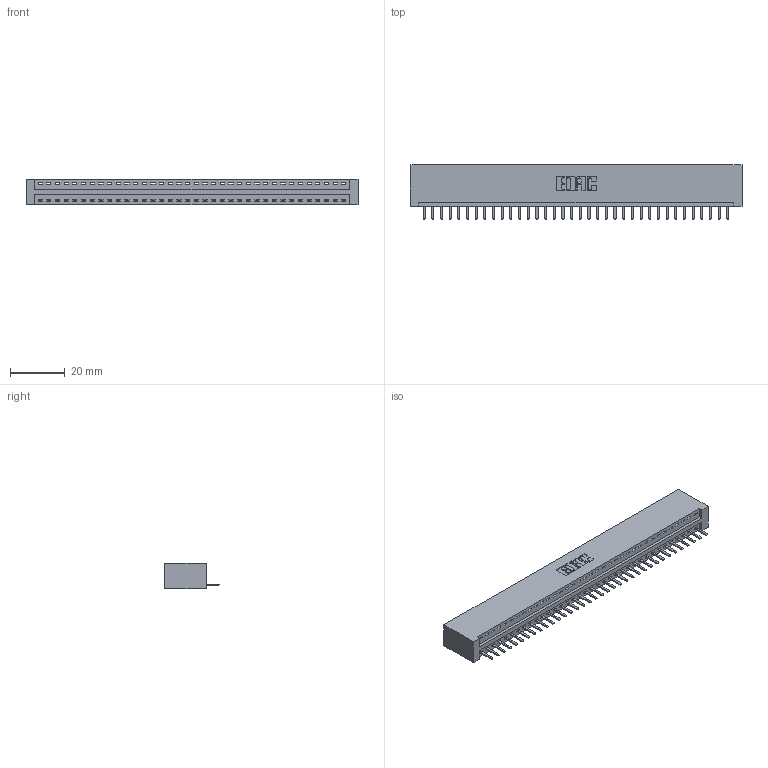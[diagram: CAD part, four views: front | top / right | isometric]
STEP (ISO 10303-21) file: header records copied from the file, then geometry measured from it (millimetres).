
FILE_DESCRIPTION (( 'STEP AP203' ), '1' );
FILE_NAME ('396-036-520-101.STEP', '2019-10-27T16:39:52', ( '' ), ( '' ), 'SwSTEP 2.0', 'SolidWorks 2016', '' );
FILE_SCHEMA (( 'CONFIG_CONTROL_DESIGN' ));
Length unit declared in the file: inch
Products named in the file (3): 346 Part_No Mounting Lugs; 396-036-520-101; 345-292-001_345-293-120
Assembly tree (37 placements, depth 2):
  396-036-520-101
    346 Part_No Mounting Lugs
    345-292-001_345-293-120  x36
Bounding box: 121.54 x 20.02 x 9.4 mm (x, y, z)
Volume: 12038.5 mm3; surface area: 14711.2 mm2
Topology: 37 solids, 37 shells, 2346 faces, 6929 edges, 4522 vertices
Faces by surface type: plane 1584, cylinder 762
Entity records: 22987 total; most frequent: CARTESIAN_POINT 3960, ORIENTED_EDGE 3918, DIRECTION 3483, EDGE_CURVE 1959, VECTOR 1687, LINE 1687, VERTEX_POINT 1302, AXIS2_PLACEMENT_3D 898
